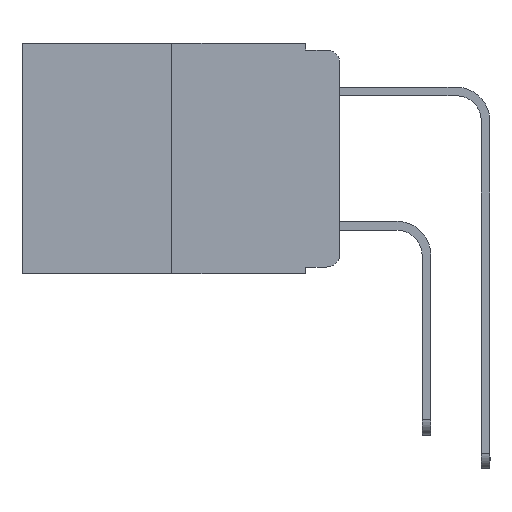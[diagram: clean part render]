
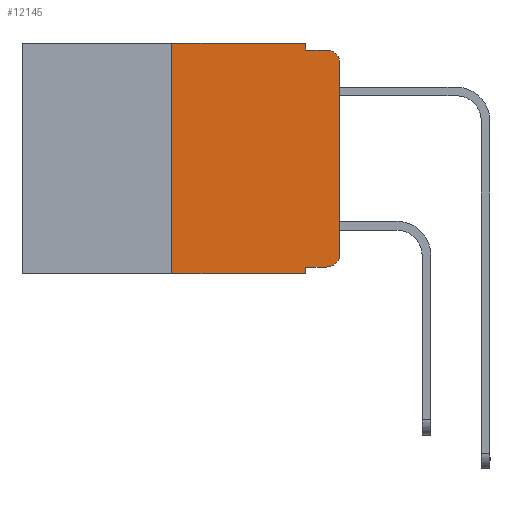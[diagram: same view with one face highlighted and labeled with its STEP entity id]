
A CAD part, left-side view. The second image highlights one B-rep face of the part: STEP entity #12145.
In plain terms, the highlighted planar face has unit normal (-1, 0, 0).
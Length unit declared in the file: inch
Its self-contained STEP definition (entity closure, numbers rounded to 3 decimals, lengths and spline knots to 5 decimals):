
#265 = VECTOR ( 'NONE', #2569, 39.37008 ) ;
#786 = EDGE_CURVE ( 'NONE', #13991, #811, #10400, .T. ) ;
#811 = VERTEX_POINT ( 'NONE', #11499 ) ;
#954 = VECTOR ( 'NONE', #2123, 39.37008 ) ;
#1318 = ORIENTED_EDGE ( 'NONE', *, *, #6341, .F. ) ;
#1323 = EDGE_CURVE ( 'NONE', #8301, #6301, #12897, .T. ) ;
#1377 = EDGE_CURVE ( 'NONE', #9864, #7806, #2279, .T. ) ;
#1679 = ORIENTED_EDGE ( 'NONE', *, *, #786, .F. ) ;
#1727 = DIRECTION ( 'NONE',  ( 0., 0., -1. ) ) ;
#1779 = ORIENTED_EDGE ( 'NONE', *, *, #13442, .F. ) ;
#2123 = DIRECTION ( 'NONE',  ( 0., 0., -1. ) ) ;
#2267 = CIRCLE ( 'NONE', #3510, 0.02 ) ;
#2279 = LINE ( 'NONE', #9600, #9436 ) ;
#2341 = LINE ( 'NONE', #3827, #265 ) ;
#2569 = DIRECTION ( 'NONE',  ( 0., -1., 0. ) ) ;
#3510 = AXIS2_PLACEMENT_3D ( 'NONE', #6871, #15252, #5670 ) ;
#3637 = VECTOR ( 'NONE', #10848, 39.37008 ) ;
#3676 = DIRECTION ( 'NONE',  ( 0., 0., 1. ) ) ;
#3683 = CARTESIAN_POINT ( 'NONE',  ( 0., 0.051, -0.343 ) ) ;
#3755 = VERTEX_POINT ( 'NONE', #8575 ) ;
#3827 = CARTESIAN_POINT ( 'NONE',  ( 0., 0.051, -0.01 ) ) ;
#3882 = LINE ( 'NONE', #8636, #14078 ) ;
#4080 = VERTEX_POINT ( 'NONE', #8478 ) ;
#4098 = ORIENTED_EDGE ( 'NONE', *, *, #5961, .T. ) ;
#4163 = ORIENTED_EDGE ( 'NONE', *, *, #14381, .F. ) ;
#4751 = CIRCLE ( 'NONE', #8735, 0.02 ) ;
#5190 = CARTESIAN_POINT ( 'NONE',  ( 0., 0.473, 0. ) ) ;
#5412 = VECTOR ( 'NONE', #7902, 39.37008 ) ;
#5580 = VERTEX_POINT ( 'NONE', #13117 ) ;
#5594 = EDGE_CURVE ( 'NONE', #5580, #6301, #3882, .T. ) ;
#5670 = DIRECTION ( 'NONE',  ( 0., 0., -1. ) ) ;
#5961 = EDGE_CURVE ( 'NONE', #8301, #3755, #7590, .T. ) ;
#5987 = DIRECTION ( 'NONE',  ( 1., 0., 0. ) ) ;
#6249 = CARTESIAN_POINT ( 'NONE',  ( 0., 0.051, 0. ) ) ;
#6301 = VERTEX_POINT ( 'NONE', #3683 ) ;
#6327 = LINE ( 'NONE', #6249, #3637 ) ;
#6341 = EDGE_CURVE ( 'NONE', #811, #4080, #6327, .T. ) ;
#6366 = FACE_OUTER_BOUND ( 'NONE', #6843, .T. ) ;
#6423 = CARTESIAN_POINT ( 'NONE',  ( 0., 0.051, -0.333 ) ) ;
#6432 = VERTEX_POINT ( 'NONE', #6638 ) ;
#6528 = CARTESIAN_POINT ( 'NONE',  ( 0., 0.25, 0. ) ) ;
#6638 = CARTESIAN_POINT ( 'NONE',  ( 0., 0.02, -0.01 ) ) ;
#6639 = DIRECTION ( 'NONE',  ( -1., 0., 0. ) ) ;
#6843 = EDGE_LOOP ( 'NONE', ( #10822, #10897, #1779, #1318, #1679, #4163, #14393, #14458, #4098, #7169 ) ) ;
#6871 = CARTESIAN_POINT ( 'NONE',  ( 0., 0.02, -0.03 ) ) ;
#7022 = PLANE ( 'NONE',  #9447 ) ;
#7053 = CARTESIAN_POINT ( 'NONE',  ( 0., 0.473, 0. ) ) ;
#7169 = ORIENTED_EDGE ( 'NONE', *, *, #14472, .T. ) ;
#7590 = LINE ( 'NONE', #6423, #7593 ) ;
#7593 = VECTOR ( 'NONE', #10946, 39.37008 ) ;
#7729 = CARTESIAN_POINT ( 'NONE',  ( 0., 0.25, 0. ) ) ;
#7806 = VERTEX_POINT ( 'NONE', #11766 ) ;
#7902 = DIRECTION ( 'NONE',  ( 0., -1., 0. ) ) ;
#8301 = VERTEX_POINT ( 'NONE', #13792 ) ;
#8478 = CARTESIAN_POINT ( 'NONE',  ( 0., 0.051, -0.01 ) ) ;
#8575 = CARTESIAN_POINT ( 'NONE',  ( 0., 0.02, -0.333 ) ) ;
#8636 = CARTESIAN_POINT ( 'NONE',  ( 0., 0.473, -0.343 ) ) ;
#8735 = AXIS2_PLACEMENT_3D ( 'NONE', #12349, #6639, #1727 ) ;
#8924 = CARTESIAN_POINT ( 'NONE',  ( 0., 0., -0.313 ) ) ;
#9436 = VECTOR ( 'NONE', #3676, 39.37008 ) ;
#9447 = AXIS2_PLACEMENT_3D ( 'NONE', #5190, #5987, #9944 ) ;
#9600 = CARTESIAN_POINT ( 'NONE',  ( 0., 0., 0. ) ) ;
#9864 = VERTEX_POINT ( 'NONE', #8924 ) ;
#9944 = DIRECTION ( 'NONE',  ( 0., 0., -1. ) ) ;
#10400 = LINE ( 'NONE', #7053, #5412 ) ;
#10822 = ORIENTED_EDGE ( 'NONE', *, *, #1377, .T. ) ;
#10848 = DIRECTION ( 'NONE',  ( 0., 0., -1. ) ) ;
#10897 = ORIENTED_EDGE ( 'NONE', *, *, #14605, .T. ) ;
#10946 = DIRECTION ( 'NONE',  ( 0., -1., 0. ) ) ;
#11499 = CARTESIAN_POINT ( 'NONE',  ( 0., 0.051, 0. ) ) ;
#11766 = CARTESIAN_POINT ( 'NONE',  ( 0., 0., -0.03 ) ) ;
#12145 = ADVANCED_FACE ( 'NONE', ( #6366 ), #7022, .F. ) ;
#12349 = CARTESIAN_POINT ( 'NONE',  ( 0., 0.02, -0.313 ) ) ;
#12648 = LINE ( 'NONE', #7729, #12724 ) ;
#12724 = VECTOR ( 'NONE', #15005, 39.37008 ) ;
#12819 = CARTESIAN_POINT ( 'NONE',  ( 0., 0.051, 0. ) ) ;
#12897 = LINE ( 'NONE', #12819, #954 ) ;
#13117 = CARTESIAN_POINT ( 'NONE',  ( 0., 0.25, -0.343 ) ) ;
#13442 = EDGE_CURVE ( 'NONE', #4080, #6432, #2341, .T. ) ;
#13789 = DIRECTION ( 'NONE',  ( 0., -1., 0. ) ) ;
#13792 = CARTESIAN_POINT ( 'NONE',  ( 0., 0.051, -0.333 ) ) ;
#13991 = VERTEX_POINT ( 'NONE', #6528 ) ;
#14078 = VECTOR ( 'NONE', #13789, 39.37008 ) ;
#14381 = EDGE_CURVE ( 'NONE', #5580, #13991, #12648, .T. ) ;
#14393 = ORIENTED_EDGE ( 'NONE', *, *, #5594, .T. ) ;
#14458 = ORIENTED_EDGE ( 'NONE', *, *, #1323, .F. ) ;
#14472 = EDGE_CURVE ( 'NONE', #3755, #9864, #4751, .T. ) ;
#14605 = EDGE_CURVE ( 'NONE', #7806, #6432, #2267, .T. ) ;
#15005 = DIRECTION ( 'NONE',  ( 0., 0., 1. ) ) ;
#15252 = DIRECTION ( 'NONE',  ( -1., 0., 0. ) ) ;
